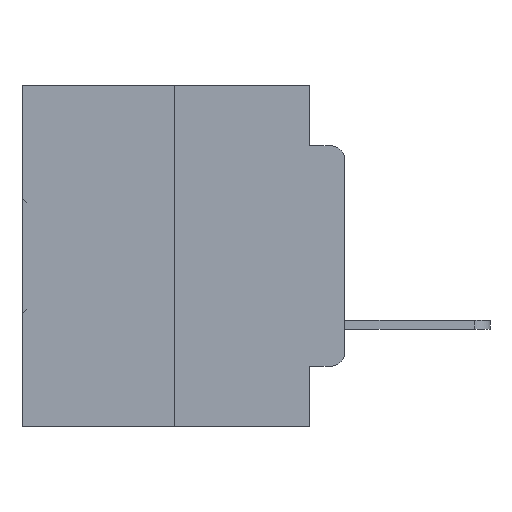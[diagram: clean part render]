
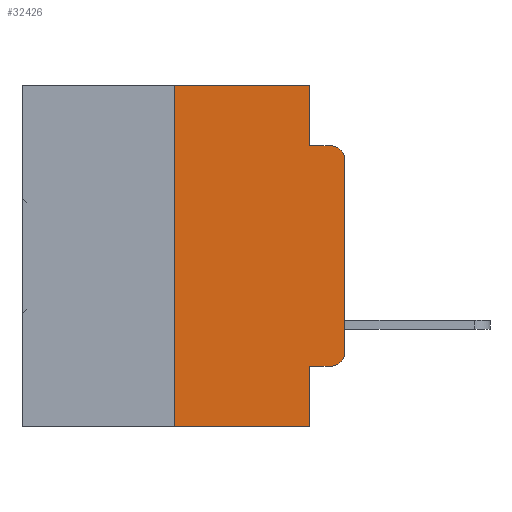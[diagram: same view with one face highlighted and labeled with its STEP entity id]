
A CAD part, left-side view. The second image highlights one B-rep face of the part: STEP entity #32426.
In plain terms, the highlighted planar face has unit normal (-1, 0, 0).
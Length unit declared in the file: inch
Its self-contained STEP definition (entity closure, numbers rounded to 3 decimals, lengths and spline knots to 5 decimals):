
#93 = DIRECTION ( 'NONE',  ( -1., 0., 0. ) ) ;
#108 = CARTESIAN_POINT ( 'NONE',  ( 0., 0.051, -0.4115 ) ) ;
#166 = EDGE_CURVE ( 'NONE', #17767, #29334, #8110, .T. ) ;
#769 = VERTEX_POINT ( 'NONE', #19765 ) ;
#1149 = VECTOR ( 'NONE', #3950, 39.37008 ) ;
#1252 = EDGE_CURVE ( 'NONE', #20292, #25518, #25197, .T. ) ;
#1496 = FACE_OUTER_BOUND ( 'NONE', #7533, .T. ) ;
#2553 = CARTESIAN_POINT ( 'NONE',  ( 0., 0.051, 0. ) ) ;
#2622 = VECTOR ( 'NONE', #7588, 39.37008 ) ;
#2828 = CARTESIAN_POINT ( 'NONE',  ( 0., 0.25, 0. ) ) ;
#3288 = ORIENTED_EDGE ( 'NONE', *, *, #1252, .T. ) ;
#3528 = ORIENTED_EDGE ( 'NONE', *, *, #25672, .F. ) ;
#3780 = DIRECTION ( 'NONE',  ( 0., 0., -1. ) ) ;
#3950 = DIRECTION ( 'NONE',  ( 0., 0., 1. ) ) ;
#4191 = CARTESIAN_POINT ( 'NONE',  ( 0., 0.02, -0.1085 ) ) ;
#4748 = ORIENTED_EDGE ( 'NONE', *, *, #24965, .F. ) ;
#5349 = CIRCLE ( 'NONE', #21874, 0.02 ) ;
#5618 = EDGE_CURVE ( 'NONE', #21399, #22785, #29056, .T. ) ;
#5626 = CARTESIAN_POINT ( 'NONE',  ( 0., 0., 0. ) ) ;
#5652 = ORIENTED_EDGE ( 'NONE', *, *, #13875, .F. ) ;
#5960 = ORIENTED_EDGE ( 'NONE', *, *, #7866, .F. ) ;
#6774 = ORIENTED_EDGE ( 'NONE', *, *, #5618, .F. ) ;
#6874 = DIRECTION ( 'NONE',  ( 0., 0., -1. ) ) ;
#7210 = VECTOR ( 'NONE', #29327, 39.37008 ) ;
#7304 = ORIENTED_EDGE ( 'NONE', *, *, #7517, .T. ) ;
#7517 = EDGE_CURVE ( 'NONE', #11698, #17767, #5349, .T. ) ;
#7533 = EDGE_LOOP ( 'NONE', ( #29615, #29671, #4748, #5960, #6774, #3528, #3288, #5652, #8644, #7304 ) ) ;
#7588 = DIRECTION ( 'NONE',  ( 0., 0., -1. ) ) ;
#7866 = EDGE_CURVE ( 'NONE', #22785, #14752, #29412, .T. ) ;
#8110 = LINE ( 'NONE', #5626, #1149 ) ;
#8490 = CARTESIAN_POINT ( 'NONE',  ( 0., 0.25, -0.5 ) ) ;
#8644 = ORIENTED_EDGE ( 'NONE', *, *, #29447, .T. ) ;
#8941 = CARTESIAN_POINT ( 'NONE',  ( 0., 0.473, 0. ) ) ;
#9006 = VECTOR ( 'NONE', #30280, 39.37008 ) ;
#10403 = LINE ( 'NONE', #12842, #2622 ) ;
#10911 = VECTOR ( 'NONE', #12558, 39.37008 ) ;
#10934 = VECTOR ( 'NONE', #26466, 39.37008 ) ;
#11192 = AXIS2_PLACEMENT_3D ( 'NONE', #8941, #19386, #3780 ) ;
#11342 = CARTESIAN_POINT ( 'NONE',  ( 0., 0.051, -0.0885 ) ) ;
#11698 = VERTEX_POINT ( 'NONE', #31768 ) ;
#11853 = VECTOR ( 'NONE', #18394, 39.37008 ) ;
#12159 = CARTESIAN_POINT ( 'NONE',  ( 0., 0.051, 0. ) ) ;
#12250 = CARTESIAN_POINT ( 'NONE',  ( 0., 0., -0.3915 ) ) ;
#12558 = DIRECTION ( 'NONE',  ( 0., -1., 0. ) ) ;
#12591 = VERTEX_POINT ( 'NONE', #20507 ) ;
#12842 = CARTESIAN_POINT ( 'NONE',  ( 0., 0.051, 0. ) ) ;
#13875 = EDGE_CURVE ( 'NONE', #12591, #25518, #10403, .T. ) ;
#14153 = LINE ( 'NONE', #14527, #7210 ) ;
#14171 = CARTESIAN_POINT ( 'NONE',  ( 0., 0.051, -0.0885 ) ) ;
#14211 = PLANE ( 'NONE',  #11192 ) ;
#14527 = CARTESIAN_POINT ( 'NONE',  ( 0., 0.25, 0. ) ) ;
#14752 = VERTEX_POINT ( 'NONE', #14171 ) ;
#14888 = EDGE_CURVE ( 'NONE', #29334, #769, #26963, .T. ) ;
#15013 = CARTESIAN_POINT ( 'NONE',  ( 0., 0.473, -0.5 ) ) ;
#15769 = CARTESIAN_POINT ( 'NONE',  ( 0., 0.02, -0.3915 ) ) ;
#16311 = CARTESIAN_POINT ( 'NONE',  ( 0., 0.051, -0.5 ) ) ;
#17143 = VECTOR ( 'NONE', #29479, 39.37008 ) ;
#17767 = VERTEX_POINT ( 'NONE', #12250 ) ;
#18382 = DIRECTION ( 'NONE',  ( 0., 0., -1. ) ) ;
#18394 = DIRECTION ( 'NONE',  ( 0., -1., 0. ) ) ;
#18758 = LINE ( 'NONE', #108, #11853 ) ;
#19386 = DIRECTION ( 'NONE',  ( 1., 0., 0. ) ) ;
#19765 = CARTESIAN_POINT ( 'NONE',  ( 0., 0.02, -0.0885 ) ) ;
#20292 = VERTEX_POINT ( 'NONE', #8490 ) ;
#20507 = CARTESIAN_POINT ( 'NONE',  ( 0., 0.051, -0.4115 ) ) ;
#21399 = VERTEX_POINT ( 'NONE', #2828 ) ;
#21874 = AXIS2_PLACEMENT_3D ( 'NONE', #15769, #93, #18382 ) ;
#22315 = DIRECTION ( 'NONE',  ( -1., 0., 0. ) ) ;
#22785 = VERTEX_POINT ( 'NONE', #2553 ) ;
#24965 = EDGE_CURVE ( 'NONE', #14752, #769, #25219, .T. ) ;
#25197 = LINE ( 'NONE', #15013, #10911 ) ;
#25219 = LINE ( 'NONE', #11342, #10934 ) ;
#25507 = CARTESIAN_POINT ( 'NONE',  ( 0., 0.473, 0. ) ) ;
#25518 = VERTEX_POINT ( 'NONE', #16311 ) ;
#25672 = EDGE_CURVE ( 'NONE', #20292, #21399, #14153, .T. ) ;
#26049 = AXIS2_PLACEMENT_3D ( 'NONE', #4191, #22315, #6874 ) ;
#26466 = DIRECTION ( 'NONE',  ( 0., -1., 0. ) ) ;
#26963 = CIRCLE ( 'NONE', #26049, 0.02 ) ;
#29056 = LINE ( 'NONE', #25507, #9006 ) ;
#29327 = DIRECTION ( 'NONE',  ( 0., 0., 1. ) ) ;
#29334 = VERTEX_POINT ( 'NONE', #32479 ) ;
#29412 = LINE ( 'NONE', #12159, #17143 ) ;
#29447 = EDGE_CURVE ( 'NONE', #12591, #11698, #18758, .T. ) ;
#29479 = DIRECTION ( 'NONE',  ( 0., 0., -1. ) ) ;
#29615 = ORIENTED_EDGE ( 'NONE', *, *, #166, .T. ) ;
#29671 = ORIENTED_EDGE ( 'NONE', *, *, #14888, .T. ) ;
#30280 = DIRECTION ( 'NONE',  ( 0., -1., 0. ) ) ;
#31768 = CARTESIAN_POINT ( 'NONE',  ( 0., 0.02, -0.4115 ) ) ;
#32426 = ADVANCED_FACE ( 'NONE', ( #1496 ), #14211, .F. ) ;
#32479 = CARTESIAN_POINT ( 'NONE',  ( 0., 0., -0.1085 ) ) ;
